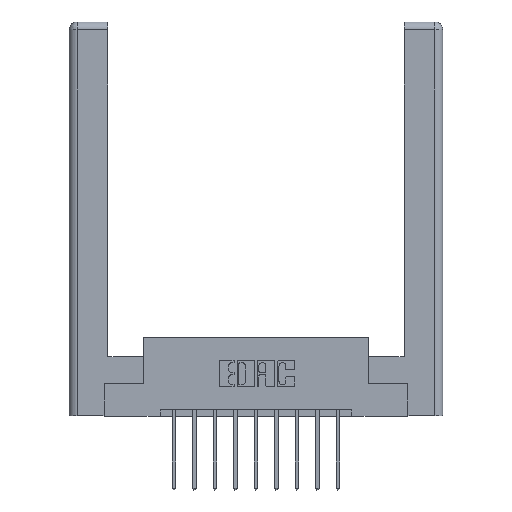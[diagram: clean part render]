
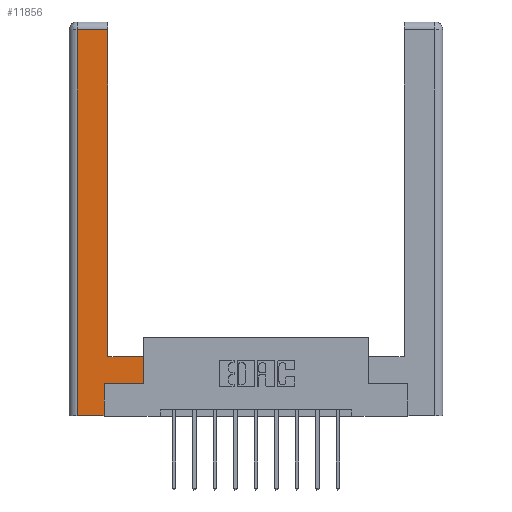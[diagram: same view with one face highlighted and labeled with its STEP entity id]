
A CAD part, top view. The second image highlights one B-rep face of the part: STEP entity #11856.
In plain terms, the highlighted planar face has unit normal (0, 0, 1).
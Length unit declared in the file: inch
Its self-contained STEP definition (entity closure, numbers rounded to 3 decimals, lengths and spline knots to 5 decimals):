
#24 = CARTESIAN_POINT ( 'NONE',  ( 0., 0., 0. ) ) ;
#186 = DIRECTION ( 'NONE',  ( 0., 1., 0. ) ) ;
#455 = EDGE_CURVE ( 'NONE', #6339, #5967, #1250, .T. ) ;
#883 = LINE ( 'NONE', #5274, #11985 ) ;
#987 = EDGE_CURVE ( 'NONE', #2244, #6339, #9338, .T. ) ;
#1092 = DIRECTION ( 'NONE',  ( -1., 0., 0. ) ) ;
#1177 = PLANE ( 'NONE',  #2646 ) ;
#1250 = LINE ( 'NONE', #12181, #4949 ) ;
#1263 = EDGE_CURVE ( 'NONE', #13059, #11696, #4265, .T. ) ;
#1358 = DIRECTION ( 'NONE',  ( 0., 1., 0. ) ) ;
#1633 = DIRECTION ( 'NONE',  ( 1., 0., 0. ) ) ;
#1750 = ORIENTED_EDGE ( 'NONE', *, *, #11183, .T. ) ;
#1969 = DIRECTION ( 'NONE',  ( 1., 0., 0. ) ) ;
#1988 = EDGE_CURVE ( 'NONE', #5967, #8023, #883, .T. ) ;
#2001 = ORIENTED_EDGE ( 'NONE', *, *, #6290, .T. ) ;
#2009 = CARTESIAN_POINT ( 'NONE',  ( 0.0615, 2.94, 0. ) ) ;
#2244 = VERTEX_POINT ( 'NONE', #13410 ) ;
#2343 = VERTEX_POINT ( 'NONE', #4814 ) ;
#2627 = VECTOR ( 'NONE', #1633, 39.37008 ) ;
#2646 = AXIS2_PLACEMENT_3D ( 'NONE', #24, #8709, #1092 ) ;
#3877 = VECTOR ( 'NONE', #7333, 39.37008 ) ;
#4204 = LINE ( 'NONE', #8557, #3877 ) ;
#4231 = LINE ( 'NONE', #10109, #5230 ) ;
#4265 = LINE ( 'NONE', #10970, #13347 ) ;
#4778 = CARTESIAN_POINT ( 'NONE',  ( 0.265, 0., 0. ) ) ;
#4814 = CARTESIAN_POINT ( 'NONE',  ( 0.565, 0.45, 0. ) ) ;
#4949 = VECTOR ( 'NONE', #186, 39.37008 ) ;
#5201 = CARTESIAN_POINT ( 'NONE',  ( 0.265, 0., 0. ) ) ;
#5230 = VECTOR ( 'NONE', #10344, 39.37008 ) ;
#5274 = CARTESIAN_POINT ( 'NONE',  ( 0.565, 0.245, 0. ) ) ;
#5299 = VECTOR ( 'NONE', #1358, 39.37008 ) ;
#5967 = VERTEX_POINT ( 'NONE', #11965 ) ;
#6290 = EDGE_CURVE ( 'NONE', #6369, #13059, #4204, .T. ) ;
#6339 = VERTEX_POINT ( 'NONE', #5201 ) ;
#6369 = VERTEX_POINT ( 'NONE', #8737 ) ;
#7333 = DIRECTION ( 'NONE',  ( 0., 1., 0. ) ) ;
#7556 = CARTESIAN_POINT ( 'NONE',  ( 0.295, 2.94, 0. ) ) ;
#8023 = VERTEX_POINT ( 'NONE', #10056 ) ;
#8438 = FACE_OUTER_BOUND ( 'NONE', #8964, .T. ) ;
#8557 = CARTESIAN_POINT ( 'NONE',  ( 0.295, 3., 0. ) ) ;
#8709 = DIRECTION ( 'NONE',  ( 0., 0., -1. ) ) ;
#8737 = CARTESIAN_POINT ( 'NONE',  ( 0.295, 0.45, 0. ) ) ;
#8754 = ORIENTED_EDGE ( 'NONE', *, *, #1263, .T. ) ;
#8890 = EDGE_CURVE ( 'NONE', #8023, #2343, #12374, .T. ) ;
#8964 = EDGE_LOOP ( 'NONE', ( #2001, #8754, #1750, #13552, #10903, #12002, #12655, #9076 ) ) ;
#9076 = ORIENTED_EDGE ( 'NONE', *, *, #11057, .T. ) ;
#9338 = LINE ( 'NONE', #4778, #2627 ) ;
#9504 = DIRECTION ( 'NONE',  ( 0., -1., 0. ) ) ;
#10056 = CARTESIAN_POINT ( 'NONE',  ( 0.565, 0.245, 0. ) ) ;
#10109 = CARTESIAN_POINT ( 'NONE',  ( 0.295, 0.45, 0. ) ) ;
#10344 = DIRECTION ( 'NONE',  ( -1., 0., 0. ) ) ;
#10903 = ORIENTED_EDGE ( 'NONE', *, *, #455, .T. ) ;
#10970 = CARTESIAN_POINT ( 'NONE',  ( 0.0615, 2.94, 0. ) ) ;
#11057 = EDGE_CURVE ( 'NONE', #2343, #6369, #4231, .T. ) ;
#11183 = EDGE_CURVE ( 'NONE', #11696, #2244, #13281, .T. ) ;
#11696 = VERTEX_POINT ( 'NONE', #2009 ) ;
#11772 = VECTOR ( 'NONE', #9504, 39.37008 ) ;
#11856 = ADVANCED_FACE ( 'NONE', ( #8438 ), #1177, .F. ) ;
#11965 = CARTESIAN_POINT ( 'NONE',  ( 0.265, 0.245, 0. ) ) ;
#11985 = VECTOR ( 'NONE', #1969, 39.37008 ) ;
#12002 = ORIENTED_EDGE ( 'NONE', *, *, #1988, .T. ) ;
#12086 = CARTESIAN_POINT ( 'NONE',  ( 0.565, 0.45, 0. ) ) ;
#12181 = CARTESIAN_POINT ( 'NONE',  ( 0.265, 0.245, 0. ) ) ;
#12374 = LINE ( 'NONE', #12086, #5299 ) ;
#12638 = CARTESIAN_POINT ( 'NONE',  ( 0.0615, 0., 0. ) ) ;
#12655 = ORIENTED_EDGE ( 'NONE', *, *, #8890, .T. ) ;
#12976 = DIRECTION ( 'NONE',  ( -1., 0., 0. ) ) ;
#13059 = VERTEX_POINT ( 'NONE', #7556 ) ;
#13281 = LINE ( 'NONE', #12638, #11772 ) ;
#13347 = VECTOR ( 'NONE', #12976, 39.37008 ) ;
#13410 = CARTESIAN_POINT ( 'NONE',  ( 0.0615, 0., 0. ) ) ;
#13552 = ORIENTED_EDGE ( 'NONE', *, *, #987, .T. ) ;
